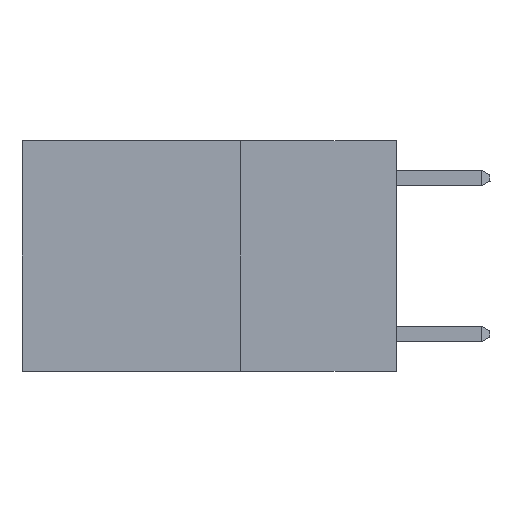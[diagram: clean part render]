
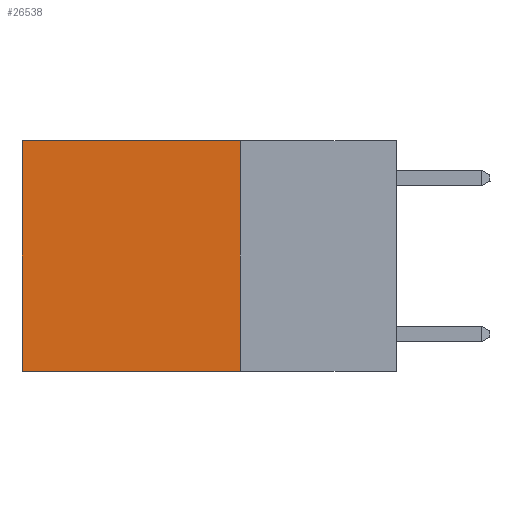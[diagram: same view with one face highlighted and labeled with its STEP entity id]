
A CAD part, left-side view. The second image highlights one B-rep face of the part: STEP entity #26538.
In plain terms, the highlighted planar face has unit normal (-1, 0, 0).
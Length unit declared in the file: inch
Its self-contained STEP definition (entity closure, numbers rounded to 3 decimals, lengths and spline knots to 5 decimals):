
#765 = EDGE_CURVE ( 'NONE', #18557, #2490, #22842, .T. ) ;
#1538 = DIRECTION ( 'NONE',  ( 0., 1., 0. ) ) ;
#1702 = PLANE ( 'NONE',  #16392 ) ;
#2490 = VERTEX_POINT ( 'NONE', #14082 ) ;
#3984 = CARTESIAN_POINT ( 'NONE',  ( 0.2625, 0.6, 0. ) ) ;
#4042 = CARTESIAN_POINT ( 'NONE',  ( 0.2625, 0.25, -0.37 ) ) ;
#6377 = ORIENTED_EDGE ( 'NONE', *, *, #15480, .F. ) ;
#7393 = VERTEX_POINT ( 'NONE', #24808 ) ;
#9469 = CARTESIAN_POINT ( 'NONE',  ( 0.2625, 0.25, 0. ) ) ;
#9961 = VECTOR ( 'NONE', #26892, 39.37008 ) ;
#10206 = VECTOR ( 'NONE', #20582, 39.37008 ) ;
#10280 = FACE_OUTER_BOUND ( 'NONE', #11197, .T. ) ;
#10424 = VECTOR ( 'NONE', #1538, 39.37008 ) ;
#11197 = EDGE_LOOP ( 'NONE', ( #19399, #6377, #14083, #23273 ) ) ;
#11262 = DIRECTION ( 'NONE',  ( 1., 0., 0. ) ) ;
#11876 = LINE ( 'NONE', #17855, #10424 ) ;
#12905 = LINE ( 'NONE', #9469, #15170 ) ;
#13362 = CARTESIAN_POINT ( 'NONE',  ( 0.2625, 0.6, 0. ) ) ;
#14082 = CARTESIAN_POINT ( 'NONE',  ( 0.2625, 0.6, -0.37 ) ) ;
#14083 = ORIENTED_EDGE ( 'NONE', *, *, #16967, .F. ) ;
#15170 = VECTOR ( 'NONE', #26498, 39.37008 ) ;
#15480 = EDGE_CURVE ( 'NONE', #19174, #2490, #11876, .T. ) ;
#16392 = AXIS2_PLACEMENT_3D ( 'NONE', #27975, #11262, #27867 ) ;
#16967 = EDGE_CURVE ( 'NONE', #7393, #19174, #12905, .T. ) ;
#17855 = CARTESIAN_POINT ( 'NONE',  ( 0.2625, 0.25, -0.37 ) ) ;
#18557 = VERTEX_POINT ( 'NONE', #3984 ) ;
#18904 = CARTESIAN_POINT ( 'NONE',  ( 0.2625, 0.25, 0. ) ) ;
#19174 = VERTEX_POINT ( 'NONE', #4042 ) ;
#19399 = ORIENTED_EDGE ( 'NONE', *, *, #765, .T. ) ;
#20582 = DIRECTION ( 'NONE',  ( 0., 0., -1. ) ) ;
#22842 = LINE ( 'NONE', #13362, #10206 ) ;
#23273 = ORIENTED_EDGE ( 'NONE', *, *, #25792, .T. ) ;
#24808 = CARTESIAN_POINT ( 'NONE',  ( 0.2625, 0.25, 0. ) ) ;
#25792 = EDGE_CURVE ( 'NONE', #7393, #18557, #29964, .T. ) ;
#26498 = DIRECTION ( 'NONE',  ( 0., 0., -1. ) ) ;
#26538 = ADVANCED_FACE ( 'NONE', ( #10280 ), #1702, .F. ) ;
#26892 = DIRECTION ( 'NONE',  ( 0., 1., 0. ) ) ;
#27867 = DIRECTION ( 'NONE',  ( 0., 0., -1. ) ) ;
#27975 = CARTESIAN_POINT ( 'NONE',  ( 0.2625, 0.25, 0. ) ) ;
#29964 = LINE ( 'NONE', #18904, #9961 ) ;
